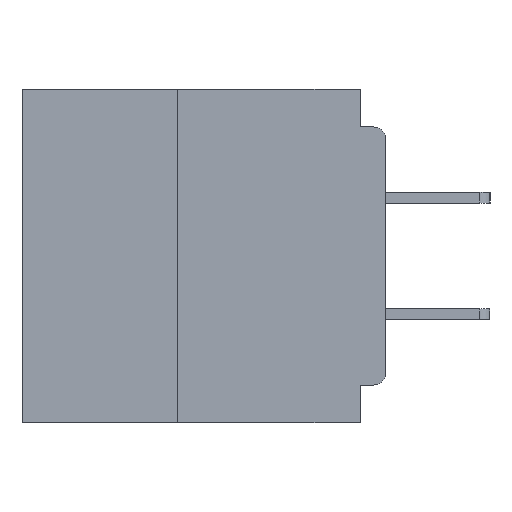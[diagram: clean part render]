
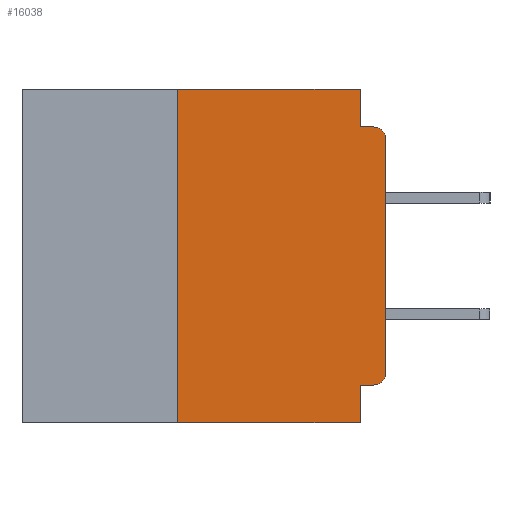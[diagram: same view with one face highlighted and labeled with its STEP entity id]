
A CAD part, left-side view. The second image highlights one B-rep face of the part: STEP entity #16038.
In plain terms, the highlighted planar face has unit normal (-1, 0, 0).
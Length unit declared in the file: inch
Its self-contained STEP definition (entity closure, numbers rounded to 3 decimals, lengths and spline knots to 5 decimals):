
#30 = CARTESIAN_POINT ( 'NONE',  ( 0., 0.437, 0. ) ) ;
#114 = ORIENTED_EDGE ( 'NONE', *, *, #2783, .T. ) ;
#716 = VERTEX_POINT ( 'NONE', #21775 ) ;
#947 = VECTOR ( 'NONE', #29470, 39.37008 ) ;
#978 = CARTESIAN_POINT ( 'NONE',  ( 0., 0.031, -0.355 ) ) ;
#1739 = CARTESIAN_POINT ( 'NONE',  ( 0., 0.437, 0. ) ) ;
#2783 = EDGE_CURVE ( 'NONE', #17726, #46891, #26236, .T. ) ;
#3204 = AXIS2_PLACEMENT_3D ( 'NONE', #42270, #18914, #46196 ) ;
#3417 = EDGE_CURVE ( 'NONE', #45435, #32959, #29913, .T. ) ;
#4034 = DIRECTION ( 'NONE',  ( 1., 0., 0. ) ) ;
#4110 = VECTOR ( 'NONE', #50910, 39.37008 ) ;
#4295 = EDGE_CURVE ( 'NONE', #716, #45435, #49300, .T. ) ;
#5144 = VECTOR ( 'NONE', #11897, 39.37008 ) ;
#5843 = EDGE_CURVE ( 'NONE', #16138, #18436, #31473, .T. ) ;
#6172 = VECTOR ( 'NONE', #7430, 39.37008 ) ;
#6820 = EDGE_CURVE ( 'NONE', #22440, #716, #28941, .T. ) ;
#6916 = LINE ( 'NONE', #9639, #16315 ) ;
#7430 = DIRECTION ( 'NONE',  ( 0., 1., 0. ) ) ;
#9639 = CARTESIAN_POINT ( 'NONE',  ( 0., 0.25, -0.4 ) ) ;
#10673 = ORIENTED_EDGE ( 'NONE', *, *, #48244, .F. ) ;
#10709 = ORIENTED_EDGE ( 'NONE', *, *, #15997, .F. ) ;
#10803 = CARTESIAN_POINT ( 'NONE',  ( 0., 0.437, -0.4 ) ) ;
#11579 = CARTESIAN_POINT ( 'NONE',  ( 0., 0.25, -0.4 ) ) ;
#11679 = ORIENTED_EDGE ( 'NONE', *, *, #5843, .F. ) ;
#11897 = DIRECTION ( 'NONE',  ( 0., -1., 0. ) ) ;
#12291 = DIRECTION ( 'NONE',  ( 0., 0., 1. ) ) ;
#12486 = ORIENTED_EDGE ( 'NONE', *, *, #6820, .T. ) ;
#13532 = LINE ( 'NONE', #47025, #4110 ) ;
#13811 = CARTESIAN_POINT ( 'NONE',  ( 0., 0.031, 0. ) ) ;
#14685 = CARTESIAN_POINT ( 'NONE',  ( 0., 0.015, -0.06 ) ) ;
#15997 = EDGE_CURVE ( 'NONE', #18436, #32959, #13532, .T. ) ;
#16038 = ADVANCED_FACE ( 'NONE', ( #22787 ), #47196, .F. ) ;
#16138 = VERTEX_POINT ( 'NONE', #28442 ) ;
#16315 = VECTOR ( 'NONE', #37149, 39.37008 ) ;
#16330 = EDGE_CURVE ( 'NONE', #31844, #16138, #50762, .T. ) ;
#16752 = ORIENTED_EDGE ( 'NONE', *, *, #21922, .F. ) ;
#17204 = CARTESIAN_POINT ( 'NONE',  ( 0., 0.25, 0. ) ) ;
#17726 = VERTEX_POINT ( 'NONE', #11579 ) ;
#18436 = VERTEX_POINT ( 'NONE', #23631 ) ;
#18582 = EDGE_LOOP ( 'NONE', ( #45180, #46163, #10709, #11679, #45490, #16752, #114, #24446, #10673, #12486 ) ) ;
#18669 = DIRECTION ( 'NONE',  ( 0., 0., -1. ) ) ;
#18697 = CARTESIAN_POINT ( 'NONE',  ( 0., 0.031, -0.4 ) ) ;
#18914 = DIRECTION ( 'NONE',  ( -1., 0., 0. ) ) ;
#19428 = VECTOR ( 'NONE', #12291, 39.37008 ) ;
#19532 = AXIS2_PLACEMENT_3D ( 'NONE', #14685, #42025, #18669 ) ;
#20062 = EDGE_CURVE ( 'NONE', #41743, #46891, #20221, .T. ) ;
#20221 = LINE ( 'NONE', #18697, #50067 ) ;
#21775 = CARTESIAN_POINT ( 'NONE',  ( 0., 0., -0.34 ) ) ;
#21922 = EDGE_CURVE ( 'NONE', #17726, #31844, #6916, .T. ) ;
#22033 = CARTESIAN_POINT ( 'NONE',  ( 0., 0., -0.06 ) ) ;
#22440 = VERTEX_POINT ( 'NONE', #43897 ) ;
#22636 = DIRECTION ( 'NONE',  ( 0., 0., -1. ) ) ;
#22787 = FACE_OUTER_BOUND ( 'NONE', #18582, .T. ) ;
#23223 = CARTESIAN_POINT ( 'NONE',  ( 0., 0., -0.355 ) ) ;
#23560 = LINE ( 'NONE', #23223, #6172 ) ;
#23631 = CARTESIAN_POINT ( 'NONE',  ( 0., 0.031, -0.045 ) ) ;
#24446 = ORIENTED_EDGE ( 'NONE', *, *, #20062, .F. ) ;
#25928 = CARTESIAN_POINT ( 'NONE',  ( 0., 0.031, -0.4 ) ) ;
#26236 = LINE ( 'NONE', #10803, #5144 ) ;
#28442 = CARTESIAN_POINT ( 'NONE',  ( 0., 0.031, 0. ) ) ;
#28941 = CIRCLE ( 'NONE', #3204, 0.015 ) ;
#29470 = DIRECTION ( 'NONE',  ( 0., -1., 0. ) ) ;
#29913 = CIRCLE ( 'NONE', #19532, 0.015 ) ;
#31473 = LINE ( 'NONE', #13811, #40621 ) ;
#31699 = DIRECTION ( 'NONE',  ( 0., 0., -1. ) ) ;
#31844 = VERTEX_POINT ( 'NONE', #17204 ) ;
#32959 = VERTEX_POINT ( 'NONE', #38349 ) ;
#37149 = DIRECTION ( 'NONE',  ( 0., 0., 1. ) ) ;
#37271 = DIRECTION ( 'NONE',  ( 0., 0., -1. ) ) ;
#38349 = CARTESIAN_POINT ( 'NONE',  ( 0., 0.015, -0.045 ) ) ;
#39718 = CARTESIAN_POINT ( 'NONE',  ( 0., 0., 0. ) ) ;
#40621 = VECTOR ( 'NONE', #37271, 39.37008 ) ;
#41743 = VERTEX_POINT ( 'NONE', #978 ) ;
#42025 = DIRECTION ( 'NONE',  ( -1., 0., 0. ) ) ;
#42270 = CARTESIAN_POINT ( 'NONE',  ( 0., 0.015, -0.34 ) ) ;
#43897 = CARTESIAN_POINT ( 'NONE',  ( 0., 0.015, -0.355 ) ) ;
#45180 = ORIENTED_EDGE ( 'NONE', *, *, #4295, .T. ) ;
#45435 = VERTEX_POINT ( 'NONE', #22033 ) ;
#45490 = ORIENTED_EDGE ( 'NONE', *, *, #16330, .F. ) ;
#46163 = ORIENTED_EDGE ( 'NONE', *, *, #3417, .T. ) ;
#46196 = DIRECTION ( 'NONE',  ( 0., 0., -1. ) ) ;
#46891 = VERTEX_POINT ( 'NONE', #25928 ) ;
#47025 = CARTESIAN_POINT ( 'NONE',  ( 0., 0., -0.045 ) ) ;
#47196 = PLANE ( 'NONE',  #47271 ) ;
#47271 = AXIS2_PLACEMENT_3D ( 'NONE', #30, #4034, #31699 ) ;
#48244 = EDGE_CURVE ( 'NONE', #22440, #41743, #23560, .T. ) ;
#49300 = LINE ( 'NONE', #39718, #19428 ) ;
#50067 = VECTOR ( 'NONE', #22636, 39.37008 ) ;
#50762 = LINE ( 'NONE', #1739, #947 ) ;
#50910 = DIRECTION ( 'NONE',  ( 0., -1., 0. ) ) ;
